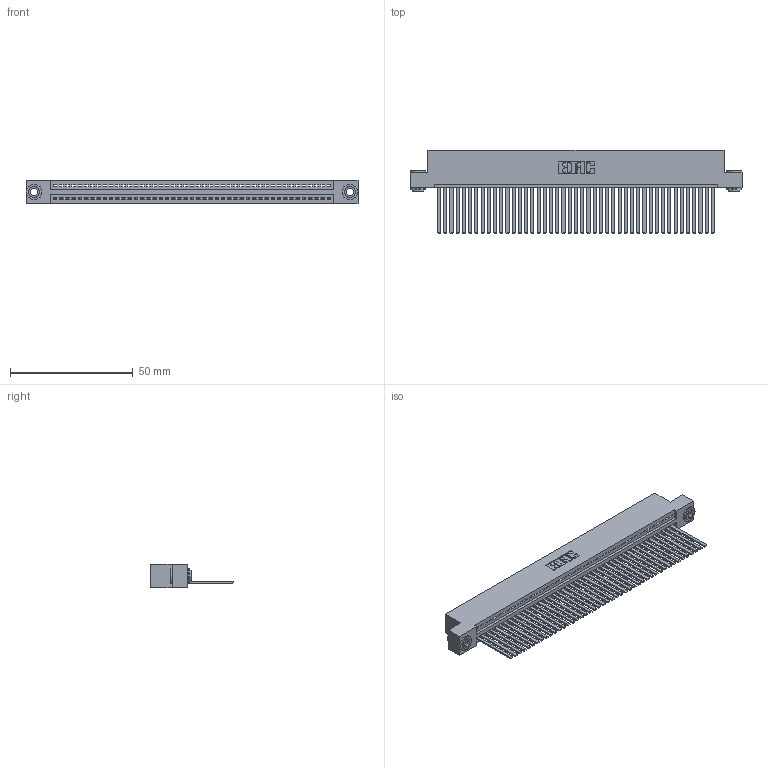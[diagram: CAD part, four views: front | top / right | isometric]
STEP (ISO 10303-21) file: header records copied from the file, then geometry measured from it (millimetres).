
FILE_DESCRIPTION (( 'STEP AP203' ), '1' );
FILE_NAME ('345-045-544-103.STEP', '2019-10-08T21:59:11', ( '' ), ( '' ), 'SwSTEP 2.0', 'SolidWorks 2016', '' );
FILE_SCHEMA (( 'CONFIG_CONTROL_DESIGN' ));
Length unit declared in the file: inch
Products named in the file (4): 345-045-544-103; 345-292-001_345-293-144; 345 Part_Flush Mounting Lugs - 0.156 Dia-TH; 345-250-002_345-250-002-102
Assembly tree (48 placements, depth 2):
  345-045-544-103
    345 Part_Flush Mounting Lugs - 0.156 Dia-TH
    345-292-001_345-293-144  x45
    345-250-002_345-250-002-102  x2
Bounding box: 135.51 x 33.96 x 9.4 mm (x, y, z)
Volume: 13435.9 mm3; surface area: 19674.9 mm2
Topology: 48 solids, 48 shells, 2504 faces, 7527 edges, 4954 vertices
Faces by surface type: plane 1710, cylinder 786, cone 8
Entity records: 33930 total; most frequent: CARTESIAN_POINT 5854, ORIENTED_EDGE 5826, DIRECTION 5137, EDGE_CURVE 2913, VECTOR 2581, LINE 2581, VERTEX_POINT 1938, AXIS2_PLACEMENT_3D 1278
